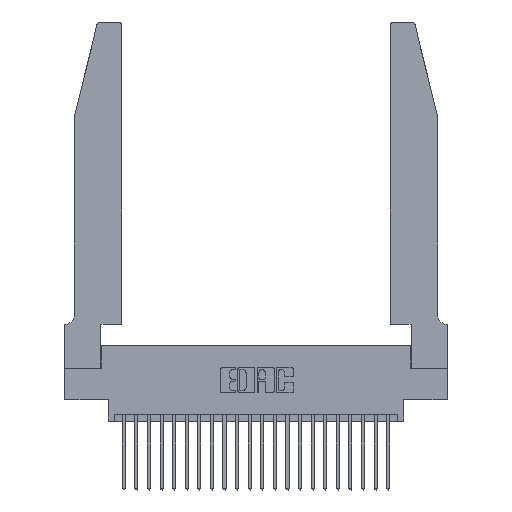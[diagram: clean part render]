
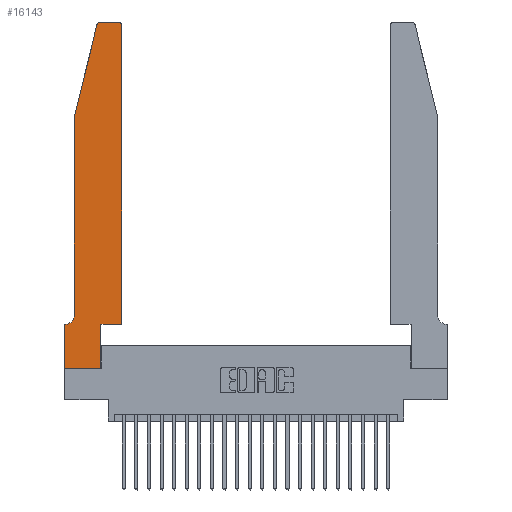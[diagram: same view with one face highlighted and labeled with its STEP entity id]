
A CAD part, top view. The second image highlights one B-rep face of the part: STEP entity #16143.
In plain terms, the highlighted planar face has unit normal (0, 0, 1).
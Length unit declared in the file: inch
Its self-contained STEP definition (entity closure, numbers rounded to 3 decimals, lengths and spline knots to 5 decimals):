
#224 = DIRECTION ( 'NONE',  ( 0., 0., 1. ) ) ;
#601 = EDGE_CURVE ( 'NONE', #13580, #22203, #4958, .T. ) ;
#682 = VECTOR ( 'NONE', #10656, 39.37008 ) ;
#794 = DIRECTION ( 'NONE',  ( 0., 0., 1. ) ) ;
#834 = CARTESIAN_POINT ( 'NONE',  ( 0.284, 2.75, 0.37 ) ) ;
#1120 = DIRECTION ( 'NONE',  ( 1., 0., 0. ) ) ;
#1305 = CARTESIAN_POINT ( 'NONE',  ( 0.25487, 2.72718, 0.37 ) ) ;
#1343 = DIRECTION ( 'NONE',  ( -0.239, -0.971, 0. ) ) ;
#1348 = ORIENTED_EDGE ( 'NONE', *, *, #2311, .T. ) ;
#1605 = LINE ( 'NONE', #14411, #682 ) ;
#1686 = EDGE_CURVE ( 'NONE', #22203, #14752, #1605, .T. ) ;
#1869 = LINE ( 'NONE', #19889, #6947 ) ;
#1979 = VECTOR ( 'NONE', #11260, 39.37008 ) ;
#2311 = EDGE_CURVE ( 'NONE', #10345, #16375, #7893, .T. ) ;
#3181 = AXIS2_PLACEMENT_3D ( 'NONE', #18029, #14413, #6638 ) ;
#3209 = CARTESIAN_POINT ( 'NONE',  ( 0.4505, 2.72, 0.37 ) ) ;
#3797 = CIRCLE ( 'NONE', #10119, 0.03 ) ;
#3927 = DIRECTION ( 'NONE',  ( 1., 0., 0. ) ) ;
#4200 = CARTESIAN_POINT ( 'NONE',  ( 0., 0., 0.37 ) ) ;
#4554 = VERTEX_POINT ( 'NONE', #3209 ) ;
#4645 = CARTESIAN_POINT ( 'NONE',  ( 0.0755, 0.35, 0.37 ) ) ;
#4958 = LINE ( 'NONE', #7208, #19975 ) ;
#5067 = CARTESIAN_POINT ( 'NONE',  ( 0., 0.35, 0.37 ) ) ;
#5468 = LINE ( 'NONE', #17935, #5778 ) ;
#5490 = ORIENTED_EDGE ( 'NONE', *, *, #9032, .T. ) ;
#5502 = DIRECTION ( 'NONE',  ( -1., 0., 0. ) ) ;
#5778 = VECTOR ( 'NONE', #21657, 39.37008 ) ;
#5797 = EDGE_CURVE ( 'NONE', #4554, #21983, #14815, .T. ) ;
#6525 = VERTEX_POINT ( 'NONE', #11452 ) ;
#6638 = DIRECTION ( 'NONE',  ( -1., 0., 0. ) ) ;
#6692 = DIRECTION ( 'NONE',  ( 1., 0., 0. ) ) ;
#6829 = VERTEX_POINT ( 'NONE', #24536 ) ;
#6947 = VECTOR ( 'NONE', #5502, 39.37008 ) ;
#7208 = CARTESIAN_POINT ( 'NONE',  ( 0.0755, 2., 0.37 ) ) ;
#7218 = EDGE_CURVE ( 'NONE', #21983, #20622, #1869, .T. ) ;
#7319 = CARTESIAN_POINT ( 'NONE',  ( 0.2865, 0.35, 0.37 ) ) ;
#7689 = CARTESIAN_POINT ( 'NONE',  ( 0.4205, 2.72, 0.37 ) ) ;
#7744 = CARTESIAN_POINT ( 'NONE',  ( 0.0755, 2., 0.37 ) ) ;
#7893 = LINE ( 'NONE', #18172, #11805 ) ;
#8657 = DIRECTION ( 'NONE',  ( 0., 0., 1. ) ) ;
#9032 = EDGE_CURVE ( 'NONE', #9470, #17036, #23411, .T. ) ;
#9470 = VERTEX_POINT ( 'NONE', #14084 ) ;
#10117 = ORIENTED_EDGE ( 'NONE', *, *, #17457, .T. ) ;
#10119 = AXIS2_PLACEMENT_3D ( 'NONE', #23874, #794, #1120 ) ;
#10345 = VERTEX_POINT ( 'NONE', #7319 ) ;
#10569 = CARTESIAN_POINT ( 'NONE',  ( 0., 0., 0.37 ) ) ;
#10656 = DIRECTION ( 'NONE',  ( 0., -1., 0. ) ) ;
#10760 = DIRECTION ( 'NONE',  ( -1., 0., 0. ) ) ;
#11260 = DIRECTION ( 'NONE',  ( 0., 1., 0. ) ) ;
#11452 = CARTESIAN_POINT ( 'NONE',  ( 0., 0., 0.37 ) ) ;
#11805 = VECTOR ( 'NONE', #6692, 39.37008 ) ;
#11811 = FACE_OUTER_BOUND ( 'NONE', #24739, .T. ) ;
#12039 = VECTOR ( 'NONE', #16095, 39.37008 ) ;
#12156 = VECTOR ( 'NONE', #12485, 39.37008 ) ;
#12221 = CARTESIAN_POINT ( 'NONE',  ( 0.4505, 0.35, 0.37 ) ) ;
#12485 = DIRECTION ( 'NONE',  ( 0., -1., 0. ) ) ;
#12902 = ORIENTED_EDGE ( 'NONE', *, *, #1686, .T. ) ;
#13215 = EDGE_CURVE ( 'NONE', #6829, #10345, #22400, .T. ) ;
#13580 = VERTEX_POINT ( 'NONE', #1305 ) ;
#13938 = ORIENTED_EDGE ( 'NONE', *, *, #13215, .T. ) ;
#14067 = ORIENTED_EDGE ( 'NONE', *, *, #21800, .T. ) ;
#14084 = CARTESIAN_POINT ( 'NONE',  ( 0.0055, 0.35, 0.37 ) ) ;
#14411 = CARTESIAN_POINT ( 'NONE',  ( 0.0755, 2., 0.37 ) ) ;
#14413 = DIRECTION ( 'NONE',  ( 0., 0., -1. ) ) ;
#14752 = VERTEX_POINT ( 'NONE', #17925 ) ;
#14765 = CARTESIAN_POINT ( 'NONE',  ( 0.4205, 2.75, 0.37 ) ) ;
#14815 = CIRCLE ( 'NONE', #23623, 0.03 ) ;
#15861 = ORIENTED_EDGE ( 'NONE', *, *, #5797, .T. ) ;
#16095 = DIRECTION ( 'NONE',  ( 1., 0., 0. ) ) ;
#16143 = ADVANCED_FACE ( 'NONE', ( #11811 ), #16446, .T. ) ;
#16208 = CARTESIAN_POINT ( 'NONE',  ( 0.2865, 0.35, 0.37 ) ) ;
#16375 = VERTEX_POINT ( 'NONE', #12221 ) ;
#16446 = PLANE ( 'NONE',  #20137 ) ;
#16555 = ORIENTED_EDGE ( 'NONE', *, *, #22462, .T. ) ;
#16601 = CARTESIAN_POINT ( 'NONE',  ( 0., 0.35, 0.37 ) ) ;
#16768 = ORIENTED_EDGE ( 'NONE', *, *, #7218, .T. ) ;
#16800 = LINE ( 'NONE', #4200, #12039 ) ;
#17036 = VERTEX_POINT ( 'NONE', #5067 ) ;
#17420 = CIRCLE ( 'NONE', #3181, 0.07 ) ;
#17457 = EDGE_CURVE ( 'NONE', #16375, #4554, #5468, .T. ) ;
#17925 = CARTESIAN_POINT ( 'NONE',  ( 0.0755, 0.42, 0.37 ) ) ;
#17935 = CARTESIAN_POINT ( 'NONE',  ( 0.4505, 0.35, 0.37 ) ) ;
#18029 = CARTESIAN_POINT ( 'NONE',  ( 0.0055, 0.42, 0.37 ) ) ;
#18171 = ORIENTED_EDGE ( 'NONE', *, *, #601, .T. ) ;
#18172 = CARTESIAN_POINT ( 'NONE',  ( 0.4505, 0.35, 0.37 ) ) ;
#19298 = EDGE_CURVE ( 'NONE', #14752, #9470, #17420, .T. ) ;
#19491 = VECTOR ( 'NONE', #10760, 39.37008 ) ;
#19671 = ORIENTED_EDGE ( 'NONE', *, *, #19298, .T. ) ;
#19889 = CARTESIAN_POINT ( 'NONE',  ( 0.2605, 2.75, 0.37 ) ) ;
#19964 = ORIENTED_EDGE ( 'NONE', *, *, #24062, .T. ) ;
#19975 = VECTOR ( 'NONE', #1343, 39.37008 ) ;
#20137 = AXIS2_PLACEMENT_3D ( 'NONE', #16601, #8657, #20146 ) ;
#20146 = DIRECTION ( 'NONE',  ( 1., 0., 0. ) ) ;
#20622 = VERTEX_POINT ( 'NONE', #834 ) ;
#21657 = DIRECTION ( 'NONE',  ( 0., 1., 0. ) ) ;
#21800 = EDGE_CURVE ( 'NONE', #20622, #13580, #3797, .T. ) ;
#21983 = VERTEX_POINT ( 'NONE', #14765 ) ;
#22074 = LINE ( 'NONE', #10569, #12156 ) ;
#22203 = VERTEX_POINT ( 'NONE', #7744 ) ;
#22400 = LINE ( 'NONE', #16208, #1979 ) ;
#22462 = EDGE_CURVE ( 'NONE', #17036, #6525, #22074, .T. ) ;
#23411 = LINE ( 'NONE', #4645, #19491 ) ;
#23623 = AXIS2_PLACEMENT_3D ( 'NONE', #7689, #224, #3927 ) ;
#23874 = CARTESIAN_POINT ( 'NONE',  ( 0.284, 2.72, 0.37 ) ) ;
#24062 = EDGE_CURVE ( 'NONE', #6525, #6829, #16800, .T. ) ;
#24536 = CARTESIAN_POINT ( 'NONE',  ( 0.2865, 0., 0.37 ) ) ;
#24739 = EDGE_LOOP ( 'NONE', ( #16768, #14067, #18171, #12902, #19671, #5490, #16555, #19964, #13938, #1348, #10117, #15861 ) ) ;
